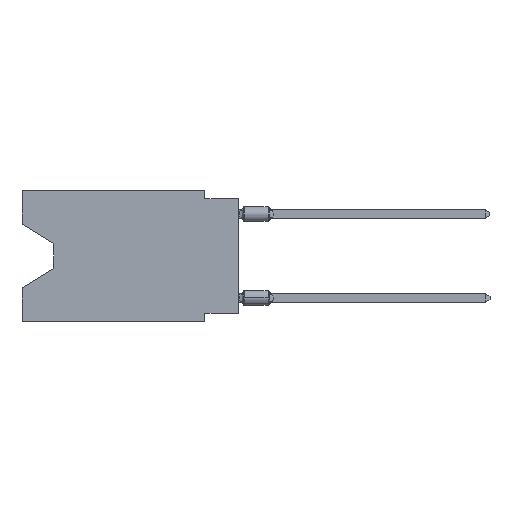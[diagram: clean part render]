
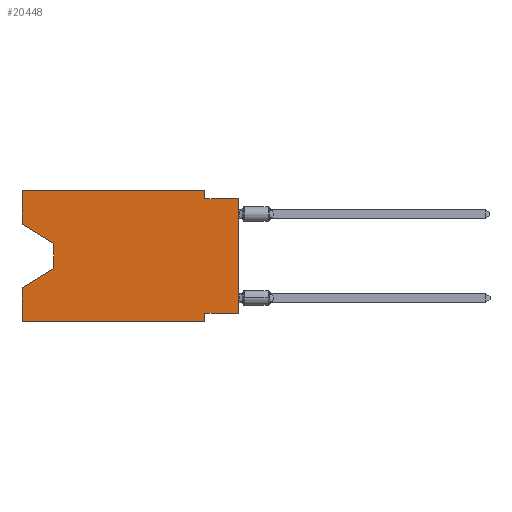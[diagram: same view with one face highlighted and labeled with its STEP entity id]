
A CAD part, left-side view. The second image highlights one B-rep face of the part: STEP entity #20448.
In plain terms, the highlighted planar face has unit normal (-1, 0, 0).
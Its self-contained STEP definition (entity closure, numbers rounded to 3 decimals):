
#143 = CARTESIAN_POINT ( 'NONE',  ( 0., 16.383, 0. ) ) ;
#150 = CARTESIAN_POINT ( 'NONE',  ( 0., 0., -9.271 ) ) ;
#335 = VECTOR ( 'NONE', #12932, 1000. ) ;
#605 = EDGE_CURVE ( 'NONE', #22359, #14662, #17186, .T. ) ;
#1072 = CARTESIAN_POINT ( 'NONE',  ( 0., 16.383, 0. ) ) ;
#1461 = VECTOR ( 'NONE', #13414, 1000. ) ;
#1667 = CARTESIAN_POINT ( 'NONE',  ( 0., 13.97, -4.013 ) ) ;
#1801 = VECTOR ( 'NONE', #6830, 1000. ) ;
#2026 = EDGE_CURVE ( 'NONE', #21754, #9152, #22356, .T. ) ;
#3333 = EDGE_CURVE ( 'NONE', #8059, #23558, #6578, .T. ) ;
#3533 = ORIENTED_EDGE ( 'NONE', *, *, #19193, .T. ) ;
#3735 = EDGE_CURVE ( 'NONE', #8059, #19575, #6680, .T. ) ;
#4029 = VECTOR ( 'NONE', #24883, 1000. ) ;
#4485 = DIRECTION ( 'NONE',  ( 0., 0., -1. ) ) ;
#4754 = FACE_OUTER_BOUND ( 'NONE', #21335, .T. ) ;
#5339 = ORIENTED_EDGE ( 'NONE', *, *, #3735, .F. ) ;
#5415 = CARTESIAN_POINT ( 'NONE',  ( 0., 0., 0. ) ) ;
#5737 = VECTOR ( 'NONE', #24968, 1000. ) ;
#5898 = ORIENTED_EDGE ( 'NONE', *, *, #17547, .F. ) ;
#6166 = CARTESIAN_POINT ( 'NONE',  ( 0., 16.383, 0. ) ) ;
#6312 = DIRECTION ( 'NONE',  ( 0., 0.855, -0.519 ) ) ;
#6463 = CARTESIAN_POINT ( 'NONE',  ( 0., 16.383, 0. ) ) ;
#6578 = LINE ( 'NONE', #18460, #9563 ) ;
#6673 = LINE ( 'NONE', #22319, #21027 ) ;
#6680 = LINE ( 'NONE', #1072, #7119 ) ;
#6693 = ORIENTED_EDGE ( 'NONE', *, *, #14060, .F. ) ;
#6749 = ORIENTED_EDGE ( 'NONE', *, *, #605, .T. ) ;
#6829 = ORIENTED_EDGE ( 'NONE', *, *, #10665, .F. ) ;
#6830 = DIRECTION ( 'NONE',  ( 0., -1., 0. ) ) ;
#7119 = VECTOR ( 'NONE', #18559, 1000. ) ;
#7300 = EDGE_CURVE ( 'NONE', #18669, #9152, #13442, .T. ) ;
#7364 = DIRECTION ( 'NONE',  ( 0., 0., 1. ) ) ;
#8059 = VERTEX_POINT ( 'NONE', #11317 ) ;
#8833 = VECTOR ( 'NONE', #17050, 1000. ) ;
#8928 = CARTESIAN_POINT ( 'NONE',  ( 0., 2.54, -9.271 ) ) ;
#9152 = VERTEX_POINT ( 'NONE', #20419 ) ;
#9563 = VECTOR ( 'NONE', #10061, 1000. ) ;
#9760 = CARTESIAN_POINT ( 'NONE',  ( 0., 2.54, -0.635 ) ) ;
#9803 = LINE ( 'NONE', #10414, #1461 ) ;
#10061 = DIRECTION ( 'NONE',  ( 0., -0.855, -0.519 ) ) ;
#10414 = CARTESIAN_POINT ( 'NONE',  ( 0., 16.383, -9.906 ) ) ;
#10620 = VERTEX_POINT ( 'NONE', #15731 ) ;
#10665 = EDGE_CURVE ( 'NONE', #19575, #10620, #23754, .T. ) ;
#11317 = CARTESIAN_POINT ( 'NONE',  ( 0., 16.383, -2.546 ) ) ;
#11465 = LINE ( 'NONE', #21182, #8833 ) ;
#12577 = CARTESIAN_POINT ( 'NONE',  ( 0., 16.383, -9.906 ) ) ;
#12656 = DIRECTION ( 'NONE',  ( 1., 0., 0. ) ) ;
#12932 = DIRECTION ( 'NONE',  ( 0., 1., 0. ) ) ;
#12969 = EDGE_CURVE ( 'NONE', #23558, #21754, #21381, .T. ) ;
#13391 = VECTOR ( 'NONE', #6312, 1000. ) ;
#13414 = DIRECTION ( 'NONE',  ( 0., -1., 0. ) ) ;
#13442 = LINE ( 'NONE', #23296, #5737 ) ;
#14060 = EDGE_CURVE ( 'NONE', #10620, #24319, #16557, .T. ) ;
#14129 = VECTOR ( 'NONE', #7364, 1000. ) ;
#14180 = CARTESIAN_POINT ( 'NONE',  ( 0., 13.97, -5.893 ) ) ;
#14343 = CARTESIAN_POINT ( 'NONE',  ( 0., 0., -9.271 ) ) ;
#14662 = VERTEX_POINT ( 'NONE', #21052 ) ;
#15430 = CARTESIAN_POINT ( 'NONE',  ( 0., 13.97, -4.013 ) ) ;
#15581 = CARTESIAN_POINT ( 'NONE',  ( 0., 2.54, -9.906 ) ) ;
#15731 = CARTESIAN_POINT ( 'NONE',  ( 0., 2.54, 0. ) ) ;
#16557 = LINE ( 'NONE', #16691, #18146 ) ;
#16603 = ORIENTED_EDGE ( 'NONE', *, *, #17151, .F. ) ;
#16691 = CARTESIAN_POINT ( 'NONE',  ( 0., 2.54, 0. ) ) ;
#16991 = VERTEX_POINT ( 'NONE', #15581 ) ;
#17050 = DIRECTION ( 'NONE',  ( 0., 0., -1. ) ) ;
#17151 = EDGE_CURVE ( 'NONE', #24319, #14662, #6673, .T. ) ;
#17186 = LINE ( 'NONE', #5415, #14129 ) ;
#17547 = EDGE_CURVE ( 'NONE', #22359, #22958, #22636, .T. ) ;
#17744 = ORIENTED_EDGE ( 'NONE', *, *, #7300, .F. ) ;
#18146 = VECTOR ( 'NONE', #18765, 1000. ) ;
#18460 = CARTESIAN_POINT ( 'NONE',  ( 0., 16.383, -2.546 ) ) ;
#18559 = DIRECTION ( 'NONE',  ( 0., 0., 1. ) ) ;
#18606 = PLANE ( 'NONE',  #25476 ) ;
#18669 = VERTEX_POINT ( 'NONE', #12577 ) ;
#18765 = DIRECTION ( 'NONE',  ( 0., 0., -1. ) ) ;
#19193 = EDGE_CURVE ( 'NONE', #18669, #16991, #9803, .T. ) ;
#19272 = ORIENTED_EDGE ( 'NONE', *, *, #2026, .T. ) ;
#19534 = ORIENTED_EDGE ( 'NONE', *, *, #3333, .T. ) ;
#19575 = VERTEX_POINT ( 'NONE', #143 ) ;
#20236 = DIRECTION ( 'NONE',  ( 0., -1., 0. ) ) ;
#20419 = CARTESIAN_POINT ( 'NONE',  ( 0., 16.383, -7.36 ) ) ;
#20448 = ADVANCED_FACE ( 'NONE', ( #4754 ), #18606, .F. ) ;
#21027 = VECTOR ( 'NONE', #20236, 1000. ) ;
#21052 = CARTESIAN_POINT ( 'NONE',  ( 0., 0., -0.635 ) ) ;
#21182 = CARTESIAN_POINT ( 'NONE',  ( 0., 2.54, -9.906 ) ) ;
#21335 = EDGE_LOOP ( 'NONE', ( #19534, #21347, #19272, #17744, #3533, #24969, #5898, #6749, #16603, #6693, #6829, #5339 ) ) ;
#21347 = ORIENTED_EDGE ( 'NONE', *, *, #12969, .T. ) ;
#21381 = LINE ( 'NONE', #15430, #4029 ) ;
#21754 = VERTEX_POINT ( 'NONE', #25318 ) ;
#22319 = CARTESIAN_POINT ( 'NONE',  ( 0., 0., -0.635 ) ) ;
#22356 = LINE ( 'NONE', #14180, #13391 ) ;
#22359 = VERTEX_POINT ( 'NONE', #150 ) ;
#22636 = LINE ( 'NONE', #14343, #335 ) ;
#22958 = VERTEX_POINT ( 'NONE', #8928 ) ;
#23296 = CARTESIAN_POINT ( 'NONE',  ( 0., 16.383, 0. ) ) ;
#23558 = VERTEX_POINT ( 'NONE', #1667 ) ;
#23754 = LINE ( 'NONE', #6166, #1801 ) ;
#24319 = VERTEX_POINT ( 'NONE', #9760 ) ;
#24883 = DIRECTION ( 'NONE',  ( 0., 0., -1. ) ) ;
#24968 = DIRECTION ( 'NONE',  ( 0., 0., 1. ) ) ;
#24969 = ORIENTED_EDGE ( 'NONE', *, *, #25535, .F. ) ;
#25318 = CARTESIAN_POINT ( 'NONE',  ( 0., 13.97, -5.893 ) ) ;
#25476 = AXIS2_PLACEMENT_3D ( 'NONE', #6463, #12656, #4485 ) ;
#25535 = EDGE_CURVE ( 'NONE', #22958, #16991, #11465, .T. ) ;
